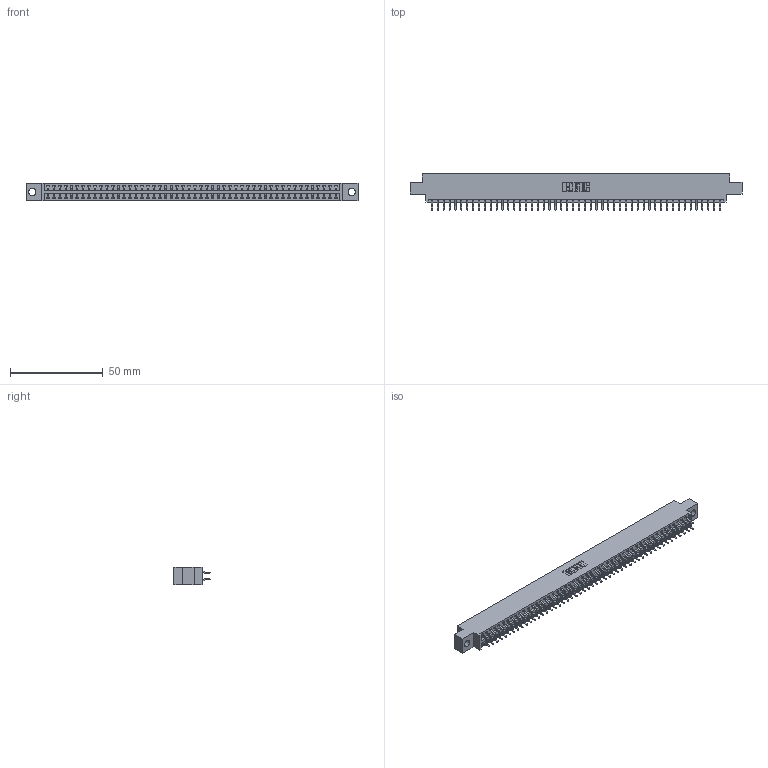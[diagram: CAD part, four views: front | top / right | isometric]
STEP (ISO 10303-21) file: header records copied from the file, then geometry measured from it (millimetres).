
FILE_DESCRIPTION (( 'STEP AP203' ), '1' );
FILE_NAME ('396-100-556-804.STEP', '2019-11-02T17:39:10', ( '' ), ( '' ), 'SwSTEP 2.0', 'SolidWorks 2016', '' );
FILE_SCHEMA (( 'CONFIG_CONTROL_DESIGN' ));
Length unit declared in the file: inch
Products named in the file (3): 346 Part_0.170 Offset - 0.156 Dia-TH; 345-292-001_556 Tail; 396-100-556-804
Assembly tree (101 placements, depth 2):
  396-100-556-804
    346 Part_0.170 Offset - 0.156 Dia-TH
    345-292-001_556 Tail  x100
Bounding box: 179.32 x 19.57 x 9.4 mm (x, y, z)
Volume: 17302 mm3; surface area: 23808.6 mm2
Topology: 101 solids, 101 shells, 5926 faces, 17641 edges, 11626 vertices
Faces by surface type: plane 3980, cylinder 1946
Entity records: 31909 total; most frequent: CARTESIAN_POINT 5264, ORIENTED_EDGE 5186, DIRECTION 4677, EDGE_CURVE 2593, LINE 2253, VECTOR 2253, VERTEX_POINT 1726, AXIS2_PLACEMENT_3D 1212
